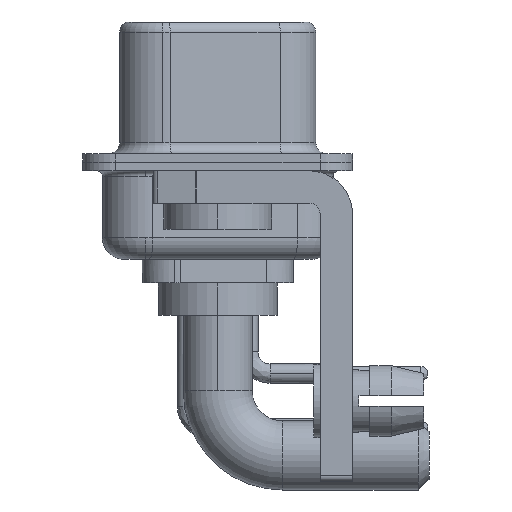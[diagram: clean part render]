
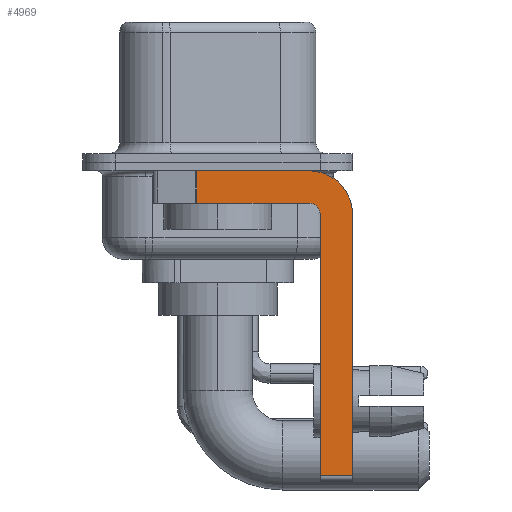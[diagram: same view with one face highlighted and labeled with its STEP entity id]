
A CAD part, left-side view. The second image highlights one B-rep face of the part: STEP entity #4969.
In plain terms, the highlighted planar face has unit normal (-1, 0, 0).
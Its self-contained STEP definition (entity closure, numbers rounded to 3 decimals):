
#311 = DIRECTION ( 'NONE',  ( 0., -1., 0. ) ) ;
#515 = FACE_OUTER_BOUND ( 'NONE', #2625, .T. ) ;
#560 = CARTESIAN_POINT ( 'NONE',  ( -2.9, -4.75, -14.8 ) ) ;
#1696 = DIRECTION ( 'NONE',  ( 0., 0., -1. ) ) ;
#2350 = EDGE_CURVE ( 'NONE', #19264, #21588, #6924, .T. ) ;
#2625 = EDGE_LOOP ( 'NONE', ( #14876, #16755, #11381, #6165, #18924, #7393, #20413, #22822 ) ) ;
#2880 = CARTESIAN_POINT ( 'NONE',  ( -2.9, -6.25, -2.4 ) ) ;
#3678 = AXIS2_PLACEMENT_3D ( 'NONE', #18318, #16418, #1696 ) ;
#3787 = AXIS2_PLACEMENT_3D ( 'NONE', #4196, #4329, #18672 ) ;
#4131 = LINE ( 'NONE', #560, #18599 ) ;
#4196 = CARTESIAN_POINT ( 'NONE',  ( -2.9, -4.25, -2.4 ) ) ;
#4329 = DIRECTION ( 'NONE',  ( 1., 0., 0. ) ) ;
#4616 = VERTEX_POINT ( 'NONE', #21585 ) ;
#4644 = AXIS2_PLACEMENT_3D ( 'NONE', #14888, #9083, #16670 ) ;
#4731 = EDGE_CURVE ( 'NONE', #8001, #11932, #11134, .T. ) ;
#4969 = ADVANCED_FACE ( 'NONE', ( #515 ), #20232, .F. ) ;
#5261 = DIRECTION ( 'NONE',  ( 0., -1., 0. ) ) ;
#5408 = DIRECTION ( 'NONE',  ( 0., 1., 0. ) ) ;
#5566 = CARTESIAN_POINT ( 'NONE',  ( -2.9, 0.978, -1.9 ) ) ;
#5681 = DIRECTION ( 'NONE',  ( 0., 0., 1. ) ) ;
#6001 = EDGE_CURVE ( 'NONE', #19264, #4616, #4131, .T. ) ;
#6165 = ORIENTED_EDGE ( 'NONE', *, *, #15032, .F. ) ;
#6830 = CARTESIAN_POINT ( 'NONE',  ( -2.9, 0.978, -1.9 ) ) ;
#6912 = CIRCLE ( 'NONE', #4644, 0.5 ) ;
#6924 = LINE ( 'NONE', #14501, #14402 ) ;
#7120 = EDGE_CURVE ( 'NONE', #8001, #11209, #10959, .T. ) ;
#7198 = CARTESIAN_POINT ( 'NONE',  ( -2.9, -6.25, -14.55 ) ) ;
#7393 = ORIENTED_EDGE ( 'NONE', *, *, #2350, .T. ) ;
#7814 = EDGE_CURVE ( 'NONE', #22342, #21588, #20409, .T. ) ;
#8001 = VERTEX_POINT ( 'NONE', #12659 ) ;
#9083 = DIRECTION ( 'NONE',  ( -1., 0., 0. ) ) ;
#9362 = CARTESIAN_POINT ( 'NONE',  ( -2.9, 3., -0.4 ) ) ;
#9606 = CARTESIAN_POINT ( 'NONE',  ( -2.9, -6.25, -2.4 ) ) ;
#9920 = VECTOR ( 'NONE', #18196, 1000. ) ;
#10959 = LINE ( 'NONE', #6830, #9920 ) ;
#11134 = LINE ( 'NONE', #9362, #14810 ) ;
#11209 = VERTEX_POINT ( 'NONE', #5566 ) ;
#11381 = ORIENTED_EDGE ( 'NONE', *, *, #15140, .F. ) ;
#11722 = DIRECTION ( 'NONE',  ( 0., 0., -1. ) ) ;
#11932 = VERTEX_POINT ( 'NONE', #15724 ) ;
#12537 = CARTESIAN_POINT ( 'NONE',  ( -2.9, -4.75, -14.55 ) ) ;
#12659 = CARTESIAN_POINT ( 'NONE',  ( -2.9, 0.978, -0.4 ) ) ;
#14402 = VECTOR ( 'NONE', #5261, 1000. ) ;
#14501 = CARTESIAN_POINT ( 'NONE',  ( -2.9, -4.25, -14.55 ) ) ;
#14810 = VECTOR ( 'NONE', #311, 1000. ) ;
#14876 = ORIENTED_EDGE ( 'NONE', *, *, #4731, .F. ) ;
#14888 = CARTESIAN_POINT ( 'NONE',  ( -2.9, -4.25, -2.4 ) ) ;
#15032 = EDGE_CURVE ( 'NONE', #4616, #19042, #6912, .T. ) ;
#15140 = EDGE_CURVE ( 'NONE', #19042, #11209, #17985, .T. ) ;
#15645 = VECTOR ( 'NONE', #11722, 1000. ) ;
#15724 = CARTESIAN_POINT ( 'NONE',  ( -2.9, -4.25, -0.4 ) ) ;
#15810 = CIRCLE ( 'NONE', #3678, 2. ) ;
#16001 = VECTOR ( 'NONE', #5408, 1000. ) ;
#16205 = CARTESIAN_POINT ( 'NONE',  ( -2.9, -4.25, -1.9 ) ) ;
#16418 = DIRECTION ( 'NONE',  ( 1., 0., 0. ) ) ;
#16670 = DIRECTION ( 'NONE',  ( 0., 0., 1. ) ) ;
#16755 = ORIENTED_EDGE ( 'NONE', *, *, #7120, .T. ) ;
#17070 = CARTESIAN_POINT ( 'NONE',  ( -2.9, -4.25, -1.9 ) ) ;
#17985 = LINE ( 'NONE', #16205, #16001 ) ;
#18196 = DIRECTION ( 'NONE',  ( 0., 0., -1. ) ) ;
#18318 = CARTESIAN_POINT ( 'NONE',  ( -2.9, -4.25, -2.4 ) ) ;
#18599 = VECTOR ( 'NONE', #5681, 1000. ) ;
#18672 = DIRECTION ( 'NONE',  ( 0., 0., -1. ) ) ;
#18924 = ORIENTED_EDGE ( 'NONE', *, *, #6001, .F. ) ;
#19042 = VERTEX_POINT ( 'NONE', #17070 ) ;
#19264 = VERTEX_POINT ( 'NONE', #12537 ) ;
#20232 = PLANE ( 'NONE',  #3787 ) ;
#20409 = LINE ( 'NONE', #9606, #15645 ) ;
#20413 = ORIENTED_EDGE ( 'NONE', *, *, #7814, .F. ) ;
#21585 = CARTESIAN_POINT ( 'NONE',  ( -2.9, -4.75, -2.4 ) ) ;
#21588 = VERTEX_POINT ( 'NONE', #7198 ) ;
#22005 = EDGE_CURVE ( 'NONE', #11932, #22342, #15810, .T. ) ;
#22342 = VERTEX_POINT ( 'NONE', #2880 ) ;
#22822 = ORIENTED_EDGE ( 'NONE', *, *, #22005, .F. ) ;
